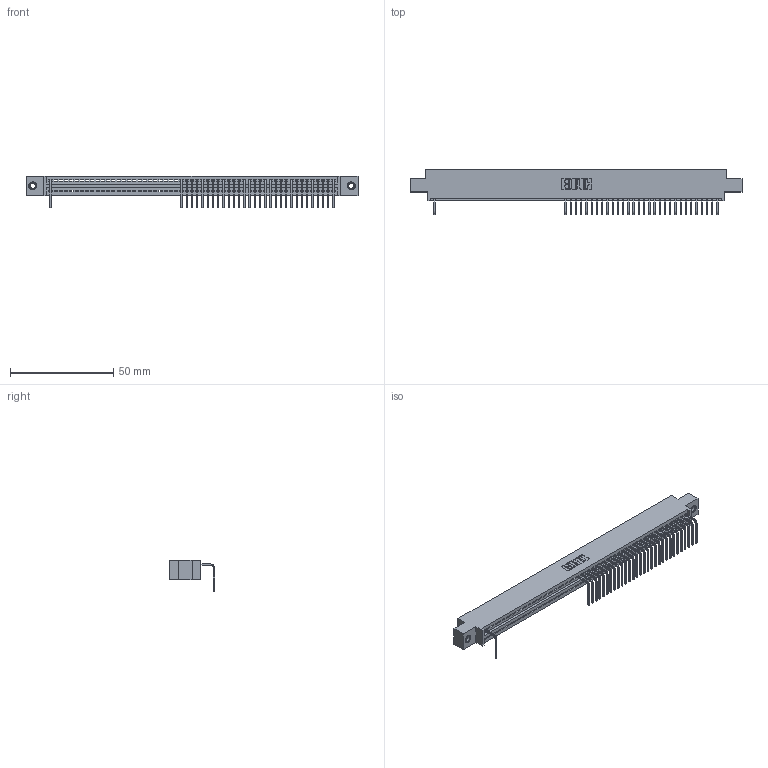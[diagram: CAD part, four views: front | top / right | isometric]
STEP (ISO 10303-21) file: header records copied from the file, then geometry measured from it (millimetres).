
FILE_DESCRIPTION (( 'STEP AP203' ), '1' );
FILE_NAME ('345-055-558-607.STEP', '2018-09-24T05:40:59', ( '' ), ( '' ), 'SwSTEP 2.0', 'SolidWorks 2016', '' );
FILE_SCHEMA (( 'CONFIG_CONTROL_DESIGN' ));
Length unit declared in the file: inch
Products named in the file (4): 345-250-001_345-250-005-103; 345-055-558-607; 345 Part_0.170 Offset - 0.156 Dia-TI; 345-292-001_558 Tail - 2
Assembly tree (34 placements, depth 2):
  345-055-558-607
    345 Part_0.170 Offset - 0.156 Dia-TI
    345-292-001_558 Tail - 2  x31
    345-250-001_345-250-005-103  x2
Bounding box: 160.91 x 21.83 x 15.37 mm (x, y, z)
Volume: 15091.4 mm3; surface area: 19538.3 mm2
Topology: 34 solids, 34 shells, 2434 faces, 7427 edges, 4902 vertices
Faces by surface type: plane 1754, cylinder 664, cone 12, torus 4
Entity records: 40278 total; most frequent: ORIENTED_EDGE 7074, CARTESIAN_POINT 7068, DIRECTION 6153, EDGE_CURVE 3537, VECTOR 3165, LINE 3165, VERTEX_POINT 2352, AXIS2_PLACEMENT_3D 1494
